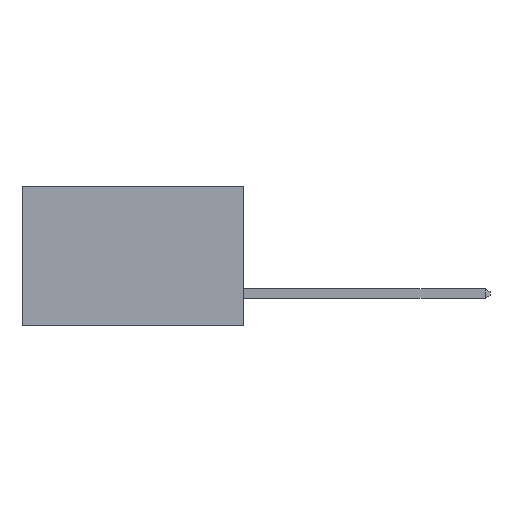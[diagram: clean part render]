
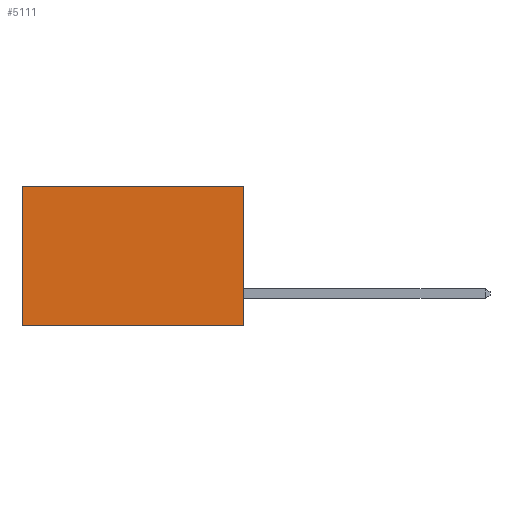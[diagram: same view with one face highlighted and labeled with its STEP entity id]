
A CAD part, left-side view. The second image highlights one B-rep face of the part: STEP entity #5111.
In plain terms, the highlighted planar face has unit normal (-1, 0, 0).
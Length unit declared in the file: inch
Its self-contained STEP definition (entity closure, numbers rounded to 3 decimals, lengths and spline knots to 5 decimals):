
#89 = DIRECTION ( 'NONE',  ( 0., 1., 0. ) ) ;
#309 = CARTESIAN_POINT ( 'NONE',  ( 0.277, 0.59, -0.37 ) ) ;
#591 = VECTOR ( 'NONE', #89, 39.37008 ) ;
#899 = VERTEX_POINT ( 'NONE', #3288 ) ;
#1014 = EDGE_CURVE ( 'NONE', #1179, #5257, #8191, .T. ) ;
#1179 = VERTEX_POINT ( 'NONE', #10144 ) ;
#1513 = EDGE_CURVE ( 'NONE', #5257, #6167, #4584, .T. ) ;
#1682 = ORIENTED_EDGE ( 'NONE', *, *, #1014, .F. ) ;
#1992 = CARTESIAN_POINT ( 'NONE',  ( 0.277, 0.59, -0.37 ) ) ;
#2030 = AXIS2_PLACEMENT_3D ( 'NONE', #8266, #8153, #8146 ) ;
#2200 = EDGE_LOOP ( 'NONE', ( #9838, #4024, #1682, #2381 ) ) ;
#2345 = DIRECTION ( 'NONE',  ( 0., 1., 0. ) ) ;
#2381 = ORIENTED_EDGE ( 'NONE', *, *, #6790, .T. ) ;
#2709 = CARTESIAN_POINT ( 'NONE',  ( 0.277, 0., -0.37 ) ) ;
#3098 = VECTOR ( 'NONE', #4644, 39.37008 ) ;
#3288 = CARTESIAN_POINT ( 'NONE',  ( 0.277, 0.59, 0. ) ) ;
#3467 = LINE ( 'NONE', #309, #3098 ) ;
#4024 = ORIENTED_EDGE ( 'NONE', *, *, #1513, .F. ) ;
#4584 = LINE ( 'NONE', #2709, #9377 ) ;
#4644 = DIRECTION ( 'NONE',  ( 0., 0., -1. ) ) ;
#5111 = ADVANCED_FACE ( 'NONE', ( #6175 ), #8198, .F. ) ;
#5257 = VERTEX_POINT ( 'NONE', #6707 ) ;
#6167 = VERTEX_POINT ( 'NONE', #1992 ) ;
#6175 = FACE_OUTER_BOUND ( 'NONE', #2200, .T. ) ;
#6388 = CARTESIAN_POINT ( 'NONE',  ( 0.277, 0., 0. ) ) ;
#6569 = LINE ( 'NONE', #6388, #591 ) ;
#6590 = DIRECTION ( 'NONE',  ( 0., 0., -1. ) ) ;
#6707 = CARTESIAN_POINT ( 'NONE',  ( 0.277, 0., -0.37 ) ) ;
#6790 = EDGE_CURVE ( 'NONE', #1179, #899, #6569, .T. ) ;
#7064 = CARTESIAN_POINT ( 'NONE',  ( 0.277, 0., -0.37 ) ) ;
#7808 = EDGE_CURVE ( 'NONE', #899, #6167, #3467, .T. ) ;
#7960 = VECTOR ( 'NONE', #6590, 39.37008 ) ;
#8146 = DIRECTION ( 'NONE',  ( 0., 0., -1. ) ) ;
#8153 = DIRECTION ( 'NONE',  ( 1., 0., 0. ) ) ;
#8191 = LINE ( 'NONE', #7064, #7960 ) ;
#8198 = PLANE ( 'NONE',  #2030 ) ;
#8266 = CARTESIAN_POINT ( 'NONE',  ( 0.277, 0., -0.37 ) ) ;
#9377 = VECTOR ( 'NONE', #2345, 39.37008 ) ;
#9838 = ORIENTED_EDGE ( 'NONE', *, *, #7808, .T. ) ;
#10144 = CARTESIAN_POINT ( 'NONE',  ( 0.277, 0., 0. ) ) ;
